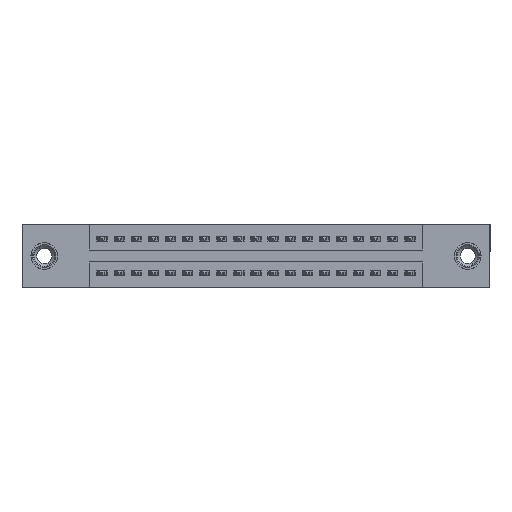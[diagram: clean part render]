
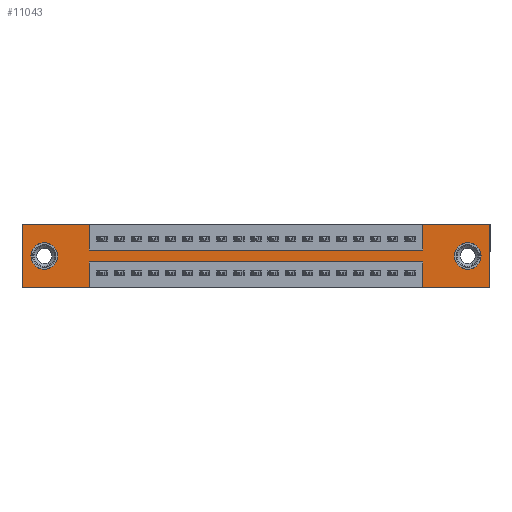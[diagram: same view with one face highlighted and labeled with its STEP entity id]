
A CAD part, front view. The second image highlights one B-rep face of the part: STEP entity #11043.
In plain terms, the highlighted planar face has unit normal (0, -1, 0).
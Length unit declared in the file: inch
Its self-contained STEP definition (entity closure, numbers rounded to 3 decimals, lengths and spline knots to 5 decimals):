
#225 = CARTESIAN_POINT ( 'NONE',  ( 0.3925, 0., 0. ) ) ;
#478 = CARTESIAN_POINT ( 'NONE',  ( 0.3925, 0., -0.22 ) ) ;
#530 = ORIENTED_EDGE ( 'NONE', *, *, #9976, .F. ) ;
#647 = EDGE_CURVE ( 'NONE', #10884, #6654, #4096, .T. ) ;
#1035 = CARTESIAN_POINT ( 'NONE',  ( 2.3425, 0., 0. ) ) ;
#1184 = CIRCLE ( 'NONE', #17253, 0.078 ) ;
#1214 = LINE ( 'NONE', #3841, #17252 ) ;
#1328 = CIRCLE ( 'NONE', #20089, 0.078 ) ;
#1444 = LINE ( 'NONE', #6150, #19686 ) ;
#1808 = CARTESIAN_POINT ( 'NONE',  ( 2.3425, 0., -0.37 ) ) ;
#1882 = DIRECTION ( 'NONE',  ( 0., 0., -1. ) ) ;
#2016 = ORIENTED_EDGE ( 'NONE', *, *, #17107, .T. ) ;
#2537 = DIRECTION ( 'NONE',  ( 0., 0., -1. ) ) ;
#2550 = FACE_BOUND ( 'NONE', #12035, .T. ) ;
#2624 = LINE ( 'NONE', #9942, #15779 ) ;
#2985 = VERTEX_POINT ( 'NONE', #12909 ) ;
#3010 = CARTESIAN_POINT ( 'NONE',  ( 0.3925, 0., -0.15 ) ) ;
#3383 = DIRECTION ( 'NONE',  ( 0., 1., 0. ) ) ;
#3526 = LINE ( 'NONE', #478, #17863 ) ;
#3558 = DIRECTION ( 'NONE',  ( 0., 1., 0. ) ) ;
#3685 = DIRECTION ( 'NONE',  ( 0., 0., -1. ) ) ;
#3841 = CARTESIAN_POINT ( 'NONE',  ( 0., 0., -0.37 ) ) ;
#4096 = LINE ( 'NONE', #16394, #15273 ) ;
#4321 = EDGE_CURVE ( 'NONE', #6654, #11590, #9998, .T. ) ;
#4322 = VECTOR ( 'NONE', #16160, 39.37008 ) ;
#4364 = CARTESIAN_POINT ( 'NONE',  ( 2.735, 0., -0.37 ) ) ;
#4640 = ORIENTED_EDGE ( 'NONE', *, *, #647, .F. ) ;
#4730 = EDGE_CURVE ( 'NONE', #14667, #18285, #16307, .T. ) ;
#4903 = EDGE_LOOP ( 'NONE', ( #10436, #18065 ) ) ;
#5477 = VERTEX_POINT ( 'NONE', #1035 ) ;
#5767 = CARTESIAN_POINT ( 'NONE',  ( 2.735, 0., 0. ) ) ;
#5953 = VERTEX_POINT ( 'NONE', #14579 ) ;
#6077 = EDGE_CURVE ( 'NONE', #18285, #19963, #2624, .T. ) ;
#6150 = CARTESIAN_POINT ( 'NONE',  ( 2.3425, 0., 0. ) ) ;
#6194 = EDGE_CURVE ( 'NONE', #5477, #14667, #16252, .T. ) ;
#6458 = DIRECTION ( 'NONE',  ( 1., 0., 0. ) ) ;
#6587 = ORIENTED_EDGE ( 'NONE', *, *, #6194, .F. ) ;
#6654 = VERTEX_POINT ( 'NONE', #225 ) ;
#6773 = CARTESIAN_POINT ( 'NONE',  ( 0.13, 0., -0.185 ) ) ;
#6942 = VECTOR ( 'NONE', #18557, 39.37008 ) ;
#7003 = EDGE_LOOP ( 'NONE', ( #8872, #15381, #530, #17064, #8672, #6587, #17628, #8243, #7096, #4640, #14886, #15339 ) ) ;
#7015 = AXIS2_PLACEMENT_3D ( 'NONE', #15549, #17490, #8570 ) ;
#7096 = ORIENTED_EDGE ( 'NONE', *, *, #4321, .F. ) ;
#7348 = DIRECTION ( 'NONE',  ( 0., 0., 1. ) ) ;
#7656 = EDGE_CURVE ( 'NONE', #12873, #5953, #19353, .T. ) ;
#8050 = CARTESIAN_POINT ( 'NONE',  ( 0., 0., -0.37 ) ) ;
#8243 = ORIENTED_EDGE ( 'NONE', *, *, #9720, .F. ) ;
#8284 = DIRECTION ( 'NONE',  ( 0., 0., 1. ) ) ;
#8430 = CARTESIAN_POINT ( 'NONE',  ( 0., 0., 0. ) ) ;
#8570 = DIRECTION ( 'NONE',  ( 0., 0., -1. ) ) ;
#8672 = ORIENTED_EDGE ( 'NONE', *, *, #4730, .F. ) ;
#8872 = ORIENTED_EDGE ( 'NONE', *, *, #7656, .F. ) ;
#8995 = DIRECTION ( 'NONE',  ( 1., 0., 0. ) ) ;
#9008 = VERTEX_POINT ( 'NONE', #18357 ) ;
#9420 = CARTESIAN_POINT ( 'NONE',  ( 0.13, 0., -0.185 ) ) ;
#9450 = EDGE_CURVE ( 'NONE', #19059, #9008, #11820, .T. ) ;
#9612 = VERTEX_POINT ( 'NONE', #19691 ) ;
#9720 = EDGE_CURVE ( 'NONE', #11590, #2985, #12325, .T. ) ;
#9917 = VERTEX_POINT ( 'NONE', #13174 ) ;
#9942 = CARTESIAN_POINT ( 'NONE',  ( 0., 0., -0.37 ) ) ;
#9976 = EDGE_CURVE ( 'NONE', #19963, #9612, #18643, .T. ) ;
#9998 = LINE ( 'NONE', #13485, #13653 ) ;
#10347 = FACE_BOUND ( 'NONE', #4903, .T. ) ;
#10399 = DIRECTION ( 'NONE',  ( -1., 0., 0. ) ) ;
#10436 = ORIENTED_EDGE ( 'NONE', *, *, #9450, .T. ) ;
#10783 = AXIS2_PLACEMENT_3D ( 'NONE', #18095, #13685, #2537 ) ;
#10884 = VERTEX_POINT ( 'NONE', #14523 ) ;
#11043 = ADVANCED_FACE ( 'NONE', ( #10347, #2550, #19107 ), #15674, .T. ) ;
#11206 = DIRECTION ( 'NONE',  ( 0., -1., 0. ) ) ;
#11590 = VERTEX_POINT ( 'NONE', #14230 ) ;
#11656 = EDGE_CURVE ( 'NONE', #9917, #17248, #1328, .T. ) ;
#11678 = LINE ( 'NONE', #8430, #15588 ) ;
#11820 = CIRCLE ( 'NONE', #7015, 0.078 ) ;
#12035 = EDGE_LOOP ( 'NONE', ( #18626, #2016 ) ) ;
#12212 = DIRECTION ( 'NONE',  ( 0., 0., 1. ) ) ;
#12325 = LINE ( 'NONE', #3010, #6942 ) ;
#12421 = CARTESIAN_POINT ( 'NONE',  ( 2.605, 0., -0.107 ) ) ;
#12765 = VECTOR ( 'NONE', #3685, 39.37008 ) ;
#12873 = VERTEX_POINT ( 'NONE', #16066 ) ;
#12909 = CARTESIAN_POINT ( 'NONE',  ( 2.3425, 0., -0.15 ) ) ;
#13006 = DIRECTION ( 'NONE',  ( -1., 0., 0. ) ) ;
#13079 = CARTESIAN_POINT ( 'NONE',  ( 0., 0., -0.37 ) ) ;
#13174 = CARTESIAN_POINT ( 'NONE',  ( 0.13, 0., -0.107 ) ) ;
#13485 = CARTESIAN_POINT ( 'NONE',  ( 0.3925, 0., 0. ) ) ;
#13653 = VECTOR ( 'NONE', #16582, 39.37008 ) ;
#13685 = DIRECTION ( 'NONE',  ( 0., 1., 0. ) ) ;
#13754 = CIRCLE ( 'NONE', #10783, 0.078 ) ;
#13885 = EDGE_CURVE ( 'NONE', #5953, #20179, #1214, .T. ) ;
#14230 = CARTESIAN_POINT ( 'NONE',  ( 0.3925, 0., -0.15 ) ) ;
#14327 = VECTOR ( 'NONE', #6458, 39.37008 ) ;
#14380 = VECTOR ( 'NONE', #16538, 39.37008 ) ;
#14523 = CARTESIAN_POINT ( 'NONE',  ( 0., 0., 0. ) ) ;
#14579 = CARTESIAN_POINT ( 'NONE',  ( 0.3925, 0., -0.37 ) ) ;
#14667 = VERTEX_POINT ( 'NONE', #15627 ) ;
#14687 = DIRECTION ( 'NONE',  ( -1., 0., 0. ) ) ;
#14886 = ORIENTED_EDGE ( 'NONE', *, *, #16229, .F. ) ;
#15273 = VECTOR ( 'NONE', #8995, 39.37008 ) ;
#15339 = ORIENTED_EDGE ( 'NONE', *, *, #13885, .F. ) ;
#15381 = ORIENTED_EDGE ( 'NONE', *, *, #15855, .F. ) ;
#15549 = CARTESIAN_POINT ( 'NONE',  ( 2.605, 0., -0.185 ) ) ;
#15588 = VECTOR ( 'NONE', #7348, 39.37008 ) ;
#15627 = CARTESIAN_POINT ( 'NONE',  ( 2.735, 0., 0. ) ) ;
#15674 = PLANE ( 'NONE',  #18747 ) ;
#15725 = CARTESIAN_POINT ( 'NONE',  ( 0., 0., 0. ) ) ;
#15779 = VECTOR ( 'NONE', #14687, 39.37008 ) ;
#15855 = EDGE_CURVE ( 'NONE', #9612, #12873, #3526, .T. ) ;
#16066 = CARTESIAN_POINT ( 'NONE',  ( 0.3925, 0., -0.22 ) ) ;
#16160 = DIRECTION ( 'NONE',  ( 0., 0., 1. ) ) ;
#16229 = EDGE_CURVE ( 'NONE', #20179, #10884, #11678, .T. ) ;
#16252 = LINE ( 'NONE', #15725, #14327 ) ;
#16298 = CARTESIAN_POINT ( 'NONE',  ( 0.3925, 0., -0.37 ) ) ;
#16307 = LINE ( 'NONE', #5767, #14380 ) ;
#16394 = CARTESIAN_POINT ( 'NONE',  ( 0., 0., 0. ) ) ;
#16538 = DIRECTION ( 'NONE',  ( 0., 0., -1. ) ) ;
#16582 = DIRECTION ( 'NONE',  ( 0., 0., -1. ) ) ;
#16896 = EDGE_CURVE ( 'NONE', #2985, #5477, #1444, .T. ) ;
#17064 = ORIENTED_EDGE ( 'NONE', *, *, #6077, .F. ) ;
#17107 = EDGE_CURVE ( 'NONE', #17248, #9917, #1184, .T. ) ;
#17248 = VERTEX_POINT ( 'NONE', #17495 ) ;
#17252 = VECTOR ( 'NONE', #10399, 39.37008 ) ;
#17253 = AXIS2_PLACEMENT_3D ( 'NONE', #9420, #3383, #19007 ) ;
#17490 = DIRECTION ( 'NONE',  ( 0., 1., 0. ) ) ;
#17495 = CARTESIAN_POINT ( 'NONE',  ( 0.13, 0., -0.263 ) ) ;
#17529 = CARTESIAN_POINT ( 'NONE',  ( 2.3425, 0., -0.37 ) ) ;
#17628 = ORIENTED_EDGE ( 'NONE', *, *, #16896, .F. ) ;
#17863 = VECTOR ( 'NONE', #13006, 39.37008 ) ;
#18065 = ORIENTED_EDGE ( 'NONE', *, *, #19408, .T. ) ;
#18095 = CARTESIAN_POINT ( 'NONE',  ( 2.605, 0., -0.185 ) ) ;
#18285 = VERTEX_POINT ( 'NONE', #4364 ) ;
#18357 = CARTESIAN_POINT ( 'NONE',  ( 2.605, 0., -0.263 ) ) ;
#18557 = DIRECTION ( 'NONE',  ( 1., 0., 0. ) ) ;
#18626 = ORIENTED_EDGE ( 'NONE', *, *, #11656, .T. ) ;
#18643 = LINE ( 'NONE', #17529, #4322 ) ;
#18747 = AXIS2_PLACEMENT_3D ( 'NONE', #8050, #11206, #1882 ) ;
#19007 = DIRECTION ( 'NONE',  ( 0., 0., 1. ) ) ;
#19059 = VERTEX_POINT ( 'NONE', #12421 ) ;
#19107 = FACE_OUTER_BOUND ( 'NONE', #7003, .T. ) ;
#19353 = LINE ( 'NONE', #16298, #12765 ) ;
#19408 = EDGE_CURVE ( 'NONE', #9008, #19059, #13754, .T. ) ;
#19686 = VECTOR ( 'NONE', #12212, 39.37008 ) ;
#19691 = CARTESIAN_POINT ( 'NONE',  ( 2.3425, 0., -0.22 ) ) ;
#19963 = VERTEX_POINT ( 'NONE', #1808 ) ;
#20089 = AXIS2_PLACEMENT_3D ( 'NONE', #6773, #3558, #8284 ) ;
#20179 = VERTEX_POINT ( 'NONE', #13079 ) ;
